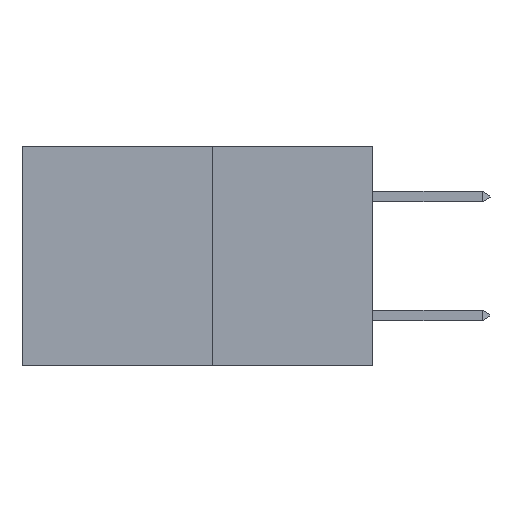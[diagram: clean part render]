
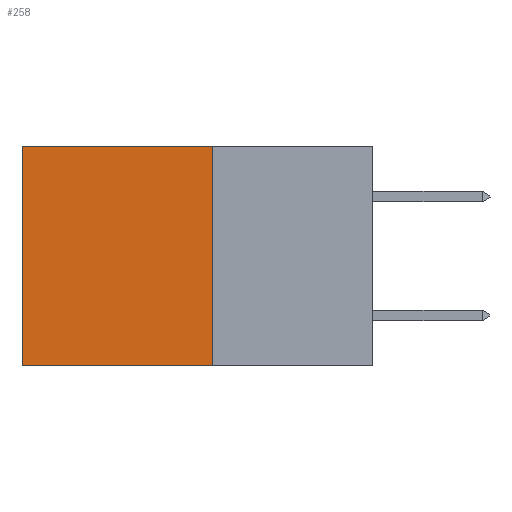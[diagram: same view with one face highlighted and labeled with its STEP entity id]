
A CAD part, left-side view. The second image highlights one B-rep face of the part: STEP entity #258.
In plain terms, the highlighted planar face has unit normal (-1, 0, 0).
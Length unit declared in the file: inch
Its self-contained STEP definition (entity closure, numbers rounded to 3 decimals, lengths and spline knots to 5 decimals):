
#217 = VECTOR ( 'NONE', #12738, 39.37008 ) ;
#258 = ADVANCED_FACE ( 'NONE', ( #5104 ), #18873, .F. ) ;
#507 = LINE ( 'NONE', #16050, #12082 ) ;
#554 = VERTEX_POINT ( 'NONE', #4304 ) ;
#801 = CARTESIAN_POINT ( 'NONE',  ( 0.277, 0.59, -0.37 ) ) ;
#1850 = CARTESIAN_POINT ( 'NONE',  ( 0.277, 0.59, -0.37 ) ) ;
#1980 = VERTEX_POINT ( 'NONE', #1850 ) ;
#2590 = DIRECTION ( 'NONE',  ( 0., 1., 0. ) ) ;
#2741 = ORIENTED_EDGE ( 'NONE', *, *, #14229, .F. ) ;
#4230 = LINE ( 'NONE', #17227, #217 ) ;
#4304 = CARTESIAN_POINT ( 'NONE',  ( 0.277, 0.27, 0. ) ) ;
#4571 = CARTESIAN_POINT ( 'NONE',  ( 0.277, 0.27, -0.37 ) ) ;
#5104 = FACE_OUTER_BOUND ( 'NONE', #10758, .T. ) ;
#6183 = CARTESIAN_POINT ( 'NONE',  ( 0.277, 0.27, -0.37 ) ) ;
#6867 = DIRECTION ( 'NONE',  ( 0., 0., -1. ) ) ;
#7373 = ORIENTED_EDGE ( 'NONE', *, *, #11410, .T. ) ;
#7756 = DIRECTION ( 'NONE',  ( 0., 0., -1. ) ) ;
#7858 = EDGE_CURVE ( 'NONE', #554, #12287, #18180, .T. ) ;
#8732 = LINE ( 'NONE', #801, #11291 ) ;
#8837 = AXIS2_PLACEMENT_3D ( 'NONE', #6183, #18900, #18921 ) ;
#9144 = CARTESIAN_POINT ( 'NONE',  ( 0.277, 0.59, 0. ) ) ;
#10758 = EDGE_LOOP ( 'NONE', ( #7373, #2741, #13886, #17949 ) ) ;
#10923 = EDGE_CURVE ( 'NONE', #554, #13744, #4230, .T. ) ;
#11291 = VECTOR ( 'NONE', #6867, 39.37008 ) ;
#11410 = EDGE_CURVE ( 'NONE', #13744, #1980, #8732, .T. ) ;
#12082 = VECTOR ( 'NONE', #2590, 39.37008 ) ;
#12287 = VERTEX_POINT ( 'NONE', #4571 ) ;
#12738 = DIRECTION ( 'NONE',  ( 0., 1., 0. ) ) ;
#13700 = CARTESIAN_POINT ( 'NONE',  ( 0.277, 0.27, -0.37 ) ) ;
#13744 = VERTEX_POINT ( 'NONE', #9144 ) ;
#13886 = ORIENTED_EDGE ( 'NONE', *, *, #7858, .F. ) ;
#14229 = EDGE_CURVE ( 'NONE', #12287, #1980, #507, .T. ) ;
#14249 = VECTOR ( 'NONE', #7756, 39.37008 ) ;
#16050 = CARTESIAN_POINT ( 'NONE',  ( 0.277, 0.27, -0.37 ) ) ;
#17227 = CARTESIAN_POINT ( 'NONE',  ( 0.277, 0.27, 0. ) ) ;
#17949 = ORIENTED_EDGE ( 'NONE', *, *, #10923, .T. ) ;
#18180 = LINE ( 'NONE', #13700, #14249 ) ;
#18873 = PLANE ( 'NONE',  #8837 ) ;
#18900 = DIRECTION ( 'NONE',  ( 1., 0., 0. ) ) ;
#18921 = DIRECTION ( 'NONE',  ( 0., 0., -1. ) ) ;
